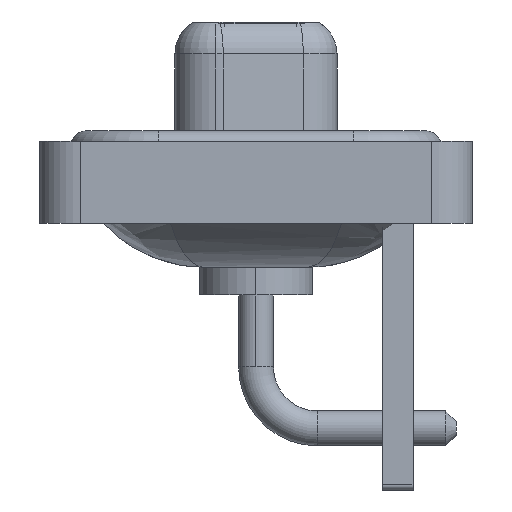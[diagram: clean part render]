
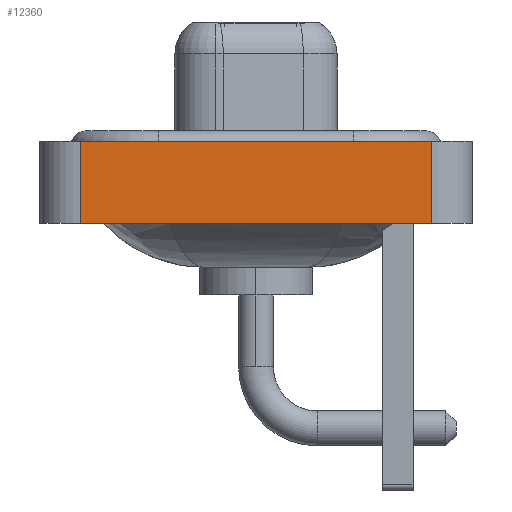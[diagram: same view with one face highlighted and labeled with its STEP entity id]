
A CAD part, left-side view. The second image highlights one B-rep face of the part: STEP entity #12360.
In plain terms, the highlighted planar face has unit normal (-1, 0, 0).
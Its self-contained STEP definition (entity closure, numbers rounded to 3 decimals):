
#471 = LINE ( 'NONE', #12620, #7159 ) ;
#618 = EDGE_CURVE ( 'NONE', #13772, #15618, #2193, .T. ) ;
#2169 = VERTEX_POINT ( 'NONE', #13224 ) ;
#2193 = LINE ( 'NONE', #15597, #5949 ) ;
#2462 = FACE_OUTER_BOUND ( 'NONE', #3883, .T. ) ;
#3252 = DIRECTION ( 'NONE',  ( 0., -1., 0. ) ) ;
#3883 = EDGE_LOOP ( 'NONE', ( #16194, #5207, #4737, #10406 ) ) ;
#4737 = ORIENTED_EDGE ( 'NONE', *, *, #15595, .F. ) ;
#4971 = DIRECTION ( 'NONE',  ( 0., 0., 1. ) ) ;
#5207 = ORIENTED_EDGE ( 'NONE', *, *, #14064, .F. ) ;
#5949 = VECTOR ( 'NONE', #7569, 1000. ) ;
#6112 = AXIS2_PLACEMENT_3D ( 'NONE', #9225, #8007, #14540 ) ;
#6472 = LINE ( 'NONE', #14499, #10637 ) ;
#7159 = VECTOR ( 'NONE', #3252, 1000. ) ;
#7186 = EDGE_CURVE ( 'NONE', #2169, #13772, #471, .T. ) ;
#7569 = DIRECTION ( 'NONE',  ( 0., 0., 1. ) ) ;
#7707 = CARTESIAN_POINT ( 'NONE',  ( -7.35, -8.55, 0.4 ) ) ;
#7806 = VERTEX_POINT ( 'NONE', #8739 ) ;
#8007 = DIRECTION ( 'NONE',  ( -1., 0., 0. ) ) ;
#8475 = LINE ( 'NONE', #15106, #9289 ) ;
#8739 = CARTESIAN_POINT ( 'NONE',  ( -7.35, 8.55, 0.4 ) ) ;
#8977 = PLANE ( 'NONE',  #6112 ) ;
#9225 = CARTESIAN_POINT ( 'NONE',  ( -7.35, -8.55, -3.6 ) ) ;
#9289 = VECTOR ( 'NONE', #9693, 1000. ) ;
#9693 = DIRECTION ( 'NONE',  ( 0., -1., 0. ) ) ;
#10406 = ORIENTED_EDGE ( 'NONE', *, *, #7186, .T. ) ;
#10637 = VECTOR ( 'NONE', #4971, 1000. ) ;
#12360 = ADVANCED_FACE ( 'NONE', ( #2462 ), #8977, .T. ) ;
#12620 = CARTESIAN_POINT ( 'NONE',  ( -7.35, -8.55, -3.6 ) ) ;
#13224 = CARTESIAN_POINT ( 'NONE',  ( -7.35, 8.55, -3.6 ) ) ;
#13772 = VERTEX_POINT ( 'NONE', #16811 ) ;
#14064 = EDGE_CURVE ( 'NONE', #7806, #15618, #8475, .T. ) ;
#14499 = CARTESIAN_POINT ( 'NONE',  ( -7.35, 8.55, -3.6 ) ) ;
#14540 = DIRECTION ( 'NONE',  ( 0., 0., 1. ) ) ;
#15106 = CARTESIAN_POINT ( 'NONE',  ( -7.35, -8.55, 0.4 ) ) ;
#15595 = EDGE_CURVE ( 'NONE', #2169, #7806, #6472, .T. ) ;
#15597 = CARTESIAN_POINT ( 'NONE',  ( -7.35, -8.55, -3.6 ) ) ;
#15618 = VERTEX_POINT ( 'NONE', #7707 ) ;
#16194 = ORIENTED_EDGE ( 'NONE', *, *, #618, .T. ) ;
#16811 = CARTESIAN_POINT ( 'NONE',  ( -7.35, -8.55, -3.6 ) ) ;
